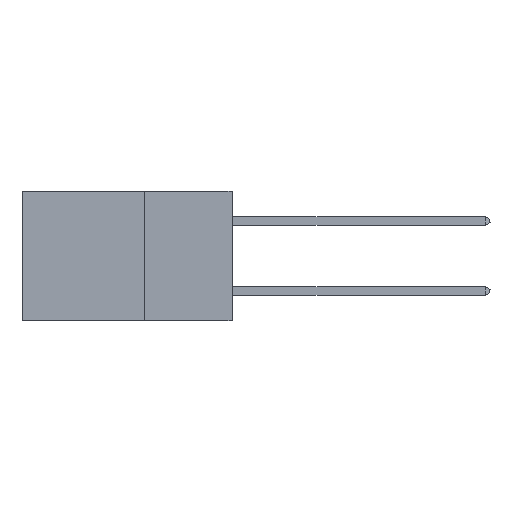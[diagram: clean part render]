
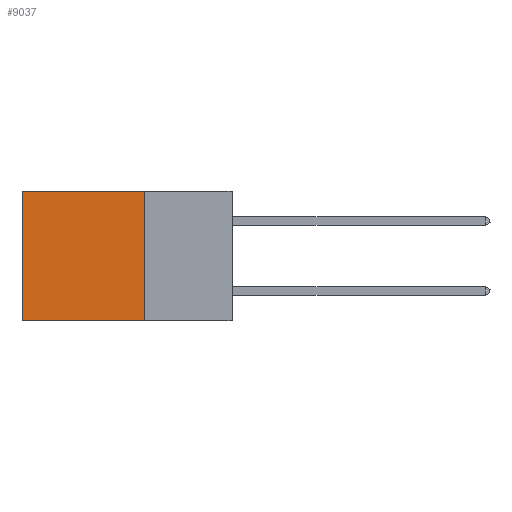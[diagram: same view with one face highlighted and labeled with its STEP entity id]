
A CAD part, left-side view. The second image highlights one B-rep face of the part: STEP entity #9037.
In plain terms, the highlighted planar face has unit normal (-1, 0, 0).
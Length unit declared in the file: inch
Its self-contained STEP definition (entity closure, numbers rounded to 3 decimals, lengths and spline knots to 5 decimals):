
#768 = DIRECTION ( 'NONE',  ( 0., 1., 0. ) ) ;
#1552 = AXIS2_PLACEMENT_3D ( 'NONE', #13826, #5806, #16849 ) ;
#2504 = PLANE ( 'NONE',  #1552 ) ;
#2524 = CARTESIAN_POINT ( 'NONE',  ( 0.2875, 0.25, 0. ) ) ;
#2590 = EDGE_CURVE ( 'NONE', #14899, #19292, #6115, .T. ) ;
#3143 = CARTESIAN_POINT ( 'NONE',  ( 0.2875, 0.25, -0.37 ) ) ;
#3424 = ORIENTED_EDGE ( 'NONE', *, *, #2590, .T. ) ;
#3481 = EDGE_CURVE ( 'NONE', #15857, #19348, #6583, .T. ) ;
#4412 = ORIENTED_EDGE ( 'NONE', *, *, #15860, .T. ) ;
#5300 = EDGE_LOOP ( 'NONE', ( #4412, #7973, #19431, #3424 ) ) ;
#5806 = DIRECTION ( 'NONE',  ( 1., 0., 0. ) ) ;
#6110 = EDGE_CURVE ( 'NONE', #14899, #15857, #6419, .T. ) ;
#6115 = LINE ( 'NONE', #19740, #18113 ) ;
#6419 = LINE ( 'NONE', #2524, #11283 ) ;
#6583 = LINE ( 'NONE', #3143, #19015 ) ;
#7058 = CARTESIAN_POINT ( 'NONE',  ( 0.2875, 0.25, -0.37 ) ) ;
#7973 = ORIENTED_EDGE ( 'NONE', *, *, #3481, .F. ) ;
#9037 = ADVANCED_FACE ( 'NONE', ( #17603 ), #2504, .F. ) ;
#9310 = VECTOR ( 'NONE', #10350, 39.37008 ) ;
#10350 = DIRECTION ( 'NONE',  ( 0., 0., -1. ) ) ;
#10696 = DIRECTION ( 'NONE',  ( 0., 0., -1. ) ) ;
#11283 = VECTOR ( 'NONE', #10696, 39.37008 ) ;
#11491 = CARTESIAN_POINT ( 'NONE',  ( 0.2875, 0.6, -0.37 ) ) ;
#13826 = CARTESIAN_POINT ( 'NONE',  ( 0.2875, 0.25, 0. ) ) ;
#14392 = DIRECTION ( 'NONE',  ( 0., 1., 0. ) ) ;
#14462 = LINE ( 'NONE', #17967, #9310 ) ;
#14899 = VERTEX_POINT ( 'NONE', #19973 ) ;
#15857 = VERTEX_POINT ( 'NONE', #7058 ) ;
#15860 = EDGE_CURVE ( 'NONE', #19292, #19348, #14462, .T. ) ;
#15973 = CARTESIAN_POINT ( 'NONE',  ( 0.2875, 0.6, 0. ) ) ;
#16849 = DIRECTION ( 'NONE',  ( 0., 0., -1. ) ) ;
#17603 = FACE_OUTER_BOUND ( 'NONE', #5300, .T. ) ;
#17967 = CARTESIAN_POINT ( 'NONE',  ( 0.2875, 0.6, 0. ) ) ;
#18113 = VECTOR ( 'NONE', #768, 39.37008 ) ;
#19015 = VECTOR ( 'NONE', #14392, 39.37008 ) ;
#19292 = VERTEX_POINT ( 'NONE', #15973 ) ;
#19348 = VERTEX_POINT ( 'NONE', #11491 ) ;
#19431 = ORIENTED_EDGE ( 'NONE', *, *, #6110, .F. ) ;
#19740 = CARTESIAN_POINT ( 'NONE',  ( 0.2875, 0.25, 0. ) ) ;
#19973 = CARTESIAN_POINT ( 'NONE',  ( 0.2875, 0.25, 0. ) ) ;
